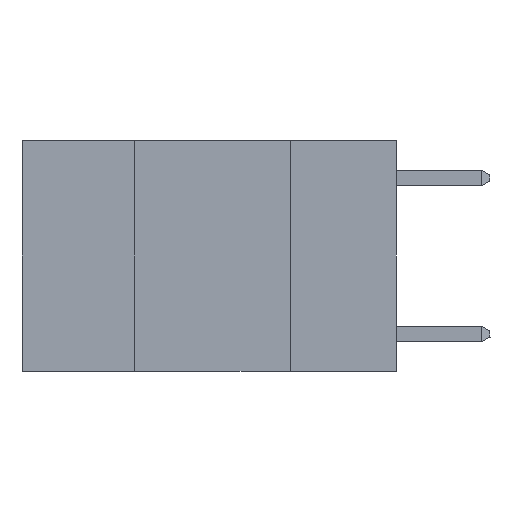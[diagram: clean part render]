
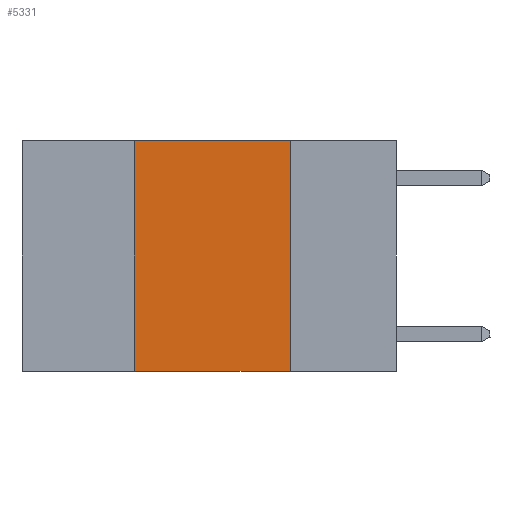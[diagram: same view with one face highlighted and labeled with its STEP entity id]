
A CAD part, left-side view. The second image highlights one B-rep face of the part: STEP entity #5331.
In plain terms, the highlighted planar face has unit normal (-1, 0, 0).
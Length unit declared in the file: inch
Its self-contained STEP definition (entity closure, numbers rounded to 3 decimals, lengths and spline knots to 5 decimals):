
#556 = CARTESIAN_POINT ( 'NONE',  ( 0., 0.42, -0.37 ) ) ;
#643 = FACE_OUTER_BOUND ( 'NONE', #8179, .T. ) ;
#740 = CARTESIAN_POINT ( 'NONE',  ( 0., 0.6, 0. ) ) ;
#742 = DIRECTION ( 'NONE',  ( 0., -1., 0. ) ) ;
#862 = VECTOR ( 'NONE', #742, 39.37008 ) ;
#1258 = ORIENTED_EDGE ( 'NONE', *, *, #4569, .F. ) ;
#1271 = ORIENTED_EDGE ( 'NONE', *, *, #2475, .F. ) ;
#1283 = ORIENTED_EDGE ( 'NONE', *, *, #3793, .F. ) ;
#1304 = ORIENTED_EDGE ( 'NONE', *, *, #5080, .T. ) ;
#1717 = AXIS2_PLACEMENT_3D ( 'NONE', #8747, #5030, #10248 ) ;
#1869 = DIRECTION ( 'NONE',  ( 0., -1., 0. ) ) ;
#1915 = DIRECTION ( 'NONE',  ( 0., 0., -1. ) ) ;
#2183 = VECTOR ( 'NONE', #1869, 39.37008 ) ;
#2351 = LINE ( 'NONE', #740, #862 ) ;
#2475 = EDGE_CURVE ( 'NONE', #8098, #7956, #2351, .T. ) ;
#3463 = CARTESIAN_POINT ( 'NONE',  ( 0., 0.6, -0.37 ) ) ;
#3793 = EDGE_CURVE ( 'NONE', #9613, #8098, #7252, .T. ) ;
#3989 = CARTESIAN_POINT ( 'NONE',  ( 0., 0.17, 0. ) ) ;
#4170 = PLANE ( 'NONE',  #1717 ) ;
#4299 = CARTESIAN_POINT ( 'NONE',  ( 0., 0.17, 0. ) ) ;
#4337 = VERTEX_POINT ( 'NONE', #5685 ) ;
#4569 = EDGE_CURVE ( 'NONE', #7956, #4337, #7578, .T. ) ;
#5030 = DIRECTION ( 'NONE',  ( 1., 0., 0. ) ) ;
#5080 = EDGE_CURVE ( 'NONE', #9613, #4337, #6432, .T. ) ;
#5331 = ADVANCED_FACE ( 'NONE', ( #643 ), #4170, .F. ) ;
#5643 = VECTOR ( 'NONE', #1915, 39.37008 ) ;
#5685 = CARTESIAN_POINT ( 'NONE',  ( 0., 0.17, -0.37 ) ) ;
#5764 = DIRECTION ( 'NONE',  ( 0., 0., 1. ) ) ;
#6432 = LINE ( 'NONE', #3463, #2183 ) ;
#6483 = CARTESIAN_POINT ( 'NONE',  ( 0., 0.42, 0. ) ) ;
#7227 = CARTESIAN_POINT ( 'NONE',  ( 0., 0.42, 0. ) ) ;
#7252 = LINE ( 'NONE', #6483, #9447 ) ;
#7578 = LINE ( 'NONE', #4299, #5643 ) ;
#7956 = VERTEX_POINT ( 'NONE', #3989 ) ;
#8098 = VERTEX_POINT ( 'NONE', #7227 ) ;
#8179 = EDGE_LOOP ( 'NONE', ( #1258, #1271, #1283, #1304 ) ) ;
#8747 = CARTESIAN_POINT ( 'NONE',  ( 0., 0.6, 0. ) ) ;
#9447 = VECTOR ( 'NONE', #5764, 39.37008 ) ;
#9613 = VERTEX_POINT ( 'NONE', #556 ) ;
#10248 = DIRECTION ( 'NONE',  ( 0., 0., -1. ) ) ;
